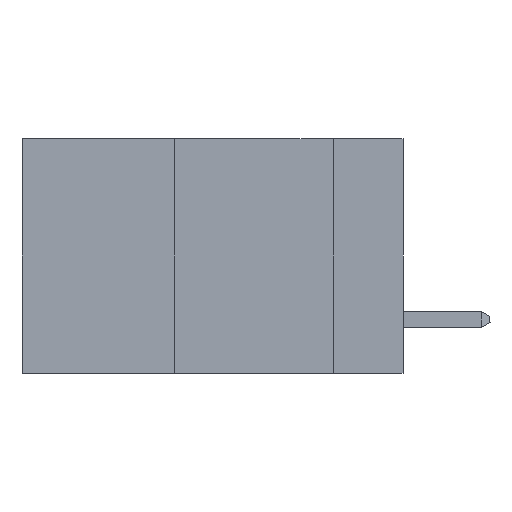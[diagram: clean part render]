
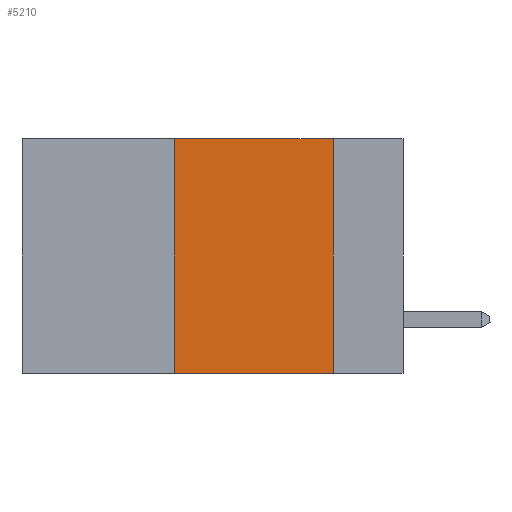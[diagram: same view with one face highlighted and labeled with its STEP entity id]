
A CAD part, left-side view. The second image highlights one B-rep face of the part: STEP entity #5210.
In plain terms, the highlighted planar face has unit normal (-1, 0, 0).
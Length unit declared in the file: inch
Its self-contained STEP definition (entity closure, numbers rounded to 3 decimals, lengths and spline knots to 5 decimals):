
#139 = VECTOR ( 'NONE', #27035, 39.37008 ) ;
#296 = EDGE_CURVE ( 'NONE', #28553, #11581, #3208, .T. ) ;
#800 = VECTOR ( 'NONE', #18085, 39.37008 ) ;
#837 = ORIENTED_EDGE ( 'NONE', *, *, #296, .F. ) ;
#866 = CARTESIAN_POINT ( 'NONE',  ( 0., 0.36, -0.37 ) ) ;
#1249 = VECTOR ( 'NONE', #32513, 39.37008 ) ;
#1321 = FACE_OUTER_BOUND ( 'NONE', #36262, .T. ) ;
#3034 = EDGE_CURVE ( 'NONE', #11581, #16352, #14909, .T. ) ;
#3208 = LINE ( 'NONE', #16514, #1249 ) ;
#3407 = VECTOR ( 'NONE', #13178, 39.37008 ) ;
#4006 = CARTESIAN_POINT ( 'NONE',  ( 0., 0.11, 0. ) ) ;
#5210 = ADVANCED_FACE ( 'NONE', ( #1321 ), #34939, .F. ) ;
#7786 = EDGE_CURVE ( 'NONE', #24652, #16352, #19197, .T. ) ;
#9595 = DIRECTION ( 'NONE',  ( 1., 0., 0. ) ) ;
#11581 = VERTEX_POINT ( 'NONE', #37072 ) ;
#13178 = DIRECTION ( 'NONE',  ( 0., 0., -1. ) ) ;
#14909 = LINE ( 'NONE', #4006, #3407 ) ;
#15577 = CARTESIAN_POINT ( 'NONE',  ( 0., 0.36, 0. ) ) ;
#16352 = VERTEX_POINT ( 'NONE', #25654 ) ;
#16514 = CARTESIAN_POINT ( 'NONE',  ( 0., 0.6, 0. ) ) ;
#18085 = DIRECTION ( 'NONE',  ( 0., -1., 0. ) ) ;
#19197 = LINE ( 'NONE', #39513, #800 ) ;
#21105 = ORIENTED_EDGE ( 'NONE', *, *, #34137, .F. ) ;
#24652 = VERTEX_POINT ( 'NONE', #866 ) ;
#25654 = CARTESIAN_POINT ( 'NONE',  ( 0., 0.11, -0.37 ) ) ;
#27035 = DIRECTION ( 'NONE',  ( 0., 0., 1. ) ) ;
#28553 = VERTEX_POINT ( 'NONE', #15577 ) ;
#29140 = ORIENTED_EDGE ( 'NONE', *, *, #7786, .T. ) ;
#31639 = DIRECTION ( 'NONE',  ( 0., 0., -1. ) ) ;
#31881 = CARTESIAN_POINT ( 'NONE',  ( 0., 0.6, 0. ) ) ;
#32513 = DIRECTION ( 'NONE',  ( 0., -1., 0. ) ) ;
#34137 = EDGE_CURVE ( 'NONE', #24652, #28553, #37307, .T. ) ;
#34939 = PLANE ( 'NONE',  #38709 ) ;
#34946 = ORIENTED_EDGE ( 'NONE', *, *, #3034, .F. ) ;
#36262 = EDGE_LOOP ( 'NONE', ( #34946, #837, #21105, #29140 ) ) ;
#36897 = CARTESIAN_POINT ( 'NONE',  ( 0., 0.36, 0. ) ) ;
#37072 = CARTESIAN_POINT ( 'NONE',  ( 0., 0.11, 0. ) ) ;
#37307 = LINE ( 'NONE', #36897, #139 ) ;
#38709 = AXIS2_PLACEMENT_3D ( 'NONE', #31881, #9595, #31639 ) ;
#39513 = CARTESIAN_POINT ( 'NONE',  ( 0., 0.6, -0.37 ) ) ;
